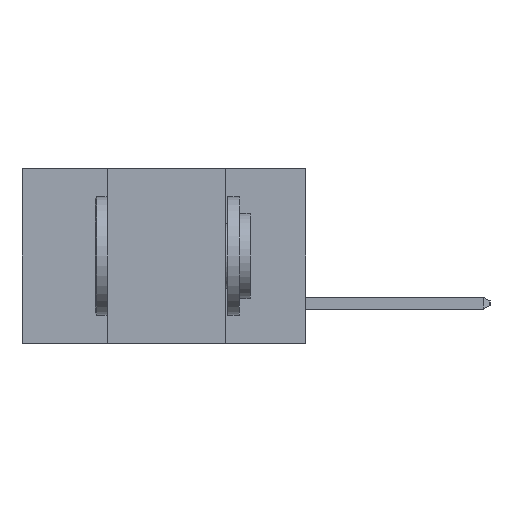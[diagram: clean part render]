
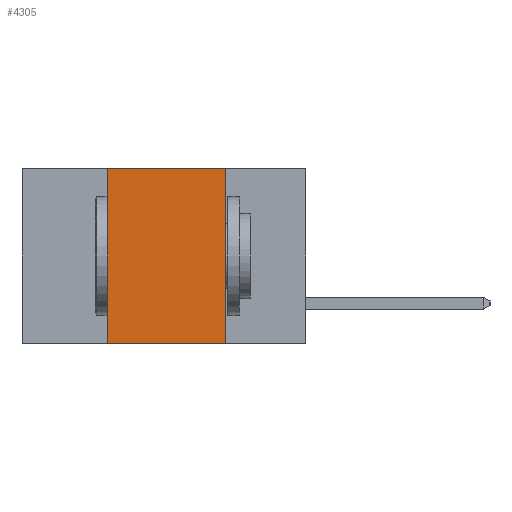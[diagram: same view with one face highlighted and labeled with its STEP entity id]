
A CAD part, left-side view. The second image highlights one B-rep face of the part: STEP entity #4305.
In plain terms, the highlighted planar face has unit normal (-1, 0, 0).
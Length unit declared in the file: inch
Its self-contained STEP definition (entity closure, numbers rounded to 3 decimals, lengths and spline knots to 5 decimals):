
#148 = DIRECTION ( 'NONE',  ( 1., 0., 0. ) ) ;
#210 = CARTESIAN_POINT ( 'NONE',  ( 0., 0.6, 0. ) ) ;
#716 = LINE ( 'NONE', #210, #4407 ) ;
#836 = LINE ( 'NONE', #7627, #4776 ) ;
#1481 = FACE_OUTER_BOUND ( 'NONE', #4412, .T. ) ;
#1712 = CARTESIAN_POINT ( 'NONE',  ( 0., 0.42, 0. ) ) ;
#1741 = EDGE_CURVE ( 'NONE', #4013, #4497, #2555, .T. ) ;
#1869 = DIRECTION ( 'NONE',  ( 0., 0., 1. ) ) ;
#2200 = PLANE ( 'NONE',  #4615 ) ;
#2335 = VECTOR ( 'NONE', #7237, 39.37008 ) ;
#2412 = ORIENTED_EDGE ( 'NONE', *, *, #1741, .F. ) ;
#2535 = ORIENTED_EDGE ( 'NONE', *, *, #4435, .F. ) ;
#2555 = LINE ( 'NONE', #8936, #2335 ) ;
#2597 = EDGE_CURVE ( 'NONE', #6840, #7089, #836, .T. ) ;
#3544 = CARTESIAN_POINT ( 'NONE',  ( 0., 0.6, 0. ) ) ;
#3797 = DIRECTION ( 'NONE',  ( 0., -1., 0. ) ) ;
#3858 = CARTESIAN_POINT ( 'NONE',  ( 0., 0.6, -0.37 ) ) ;
#4013 = VERTEX_POINT ( 'NONE', #5416 ) ;
#4305 = ADVANCED_FACE ( 'NONE', ( #1481 ), #2200, .F. ) ;
#4407 = VECTOR ( 'NONE', #9511, 39.37008 ) ;
#4412 = EDGE_LOOP ( 'NONE', ( #2412, #2535, #6070, #7342 ) ) ;
#4435 = EDGE_CURVE ( 'NONE', #7089, #4013, #716, .T. ) ;
#4497 = VERTEX_POINT ( 'NONE', #7725 ) ;
#4609 = LINE ( 'NONE', #3858, #6398 ) ;
#4615 = AXIS2_PLACEMENT_3D ( 'NONE', #3544, #148, #9623 ) ;
#4776 = VECTOR ( 'NONE', #1869, 39.37008 ) ;
#5326 = EDGE_CURVE ( 'NONE', #6840, #4497, #4609, .T. ) ;
#5416 = CARTESIAN_POINT ( 'NONE',  ( 0., 0.17, 0. ) ) ;
#6070 = ORIENTED_EDGE ( 'NONE', *, *, #2597, .F. ) ;
#6398 = VECTOR ( 'NONE', #3797, 39.37008 ) ;
#6715 = CARTESIAN_POINT ( 'NONE',  ( 0., 0.42, -0.37 ) ) ;
#6840 = VERTEX_POINT ( 'NONE', #6715 ) ;
#7089 = VERTEX_POINT ( 'NONE', #1712 ) ;
#7237 = DIRECTION ( 'NONE',  ( 0., 0., -1. ) ) ;
#7342 = ORIENTED_EDGE ( 'NONE', *, *, #5326, .T. ) ;
#7627 = CARTESIAN_POINT ( 'NONE',  ( 0., 0.42, -0.37 ) ) ;
#7725 = CARTESIAN_POINT ( 'NONE',  ( 0., 0.17, -0.37 ) ) ;
#8936 = CARTESIAN_POINT ( 'NONE',  ( 0., 0.17, -0.37 ) ) ;
#9511 = DIRECTION ( 'NONE',  ( 0., -1., 0. ) ) ;
#9623 = DIRECTION ( 'NONE',  ( 0., 0., -1. ) ) ;
